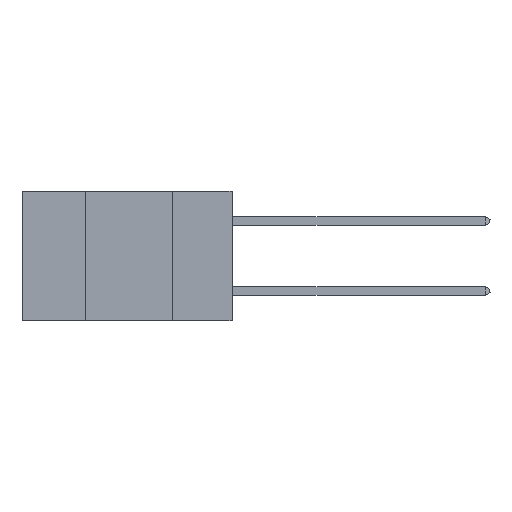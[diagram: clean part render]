
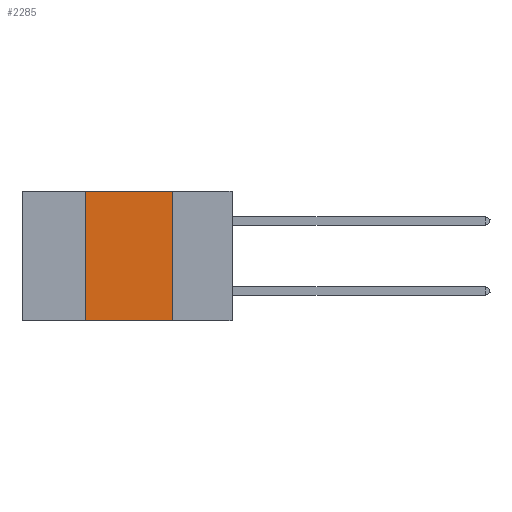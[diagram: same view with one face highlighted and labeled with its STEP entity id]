
A CAD part, left-side view. The second image highlights one B-rep face of the part: STEP entity #2285.
In plain terms, the highlighted planar face has unit normal (-1, 0, 0).
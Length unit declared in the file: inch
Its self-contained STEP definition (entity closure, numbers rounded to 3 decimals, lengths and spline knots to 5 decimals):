
#18 = CARTESIAN_POINT ( 'NONE',  ( 0., 0.6, -0.37 ) ) ;
#862 = DIRECTION ( 'NONE',  ( 0., 0., -1. ) ) ;
#1219 = FACE_OUTER_BOUND ( 'NONE', #6404, .T. ) ;
#1738 = CARTESIAN_POINT ( 'NONE',  ( 0., 0.42, -0.37 ) ) ;
#2285 = ADVANCED_FACE ( 'NONE', ( #1219 ), #3434, .F. ) ;
#2644 = EDGE_CURVE ( 'NONE', #15117, #19382, #21342, .T. ) ;
#2808 = VECTOR ( 'NONE', #862, 39.37008 ) ;
#3316 = LINE ( 'NONE', #18, #18737 ) ;
#3434 = PLANE ( 'NONE',  #4460 ) ;
#4152 = VERTEX_POINT ( 'NONE', #21878 ) ;
#4460 = AXIS2_PLACEMENT_3D ( 'NONE', #15384, #17049, #6880 ) ;
#5957 = ORIENTED_EDGE ( 'NONE', *, *, #6085, .T. ) ;
#6085 = EDGE_CURVE ( 'NONE', #17109, #19382, #3316, .T. ) ;
#6404 = EDGE_LOOP ( 'NONE', ( #21267, #8382, #13444, #5957 ) ) ;
#6756 = VECTOR ( 'NONE', #12698, 39.37008 ) ;
#6880 = DIRECTION ( 'NONE',  ( 0., 0., -1. ) ) ;
#7506 = EDGE_CURVE ( 'NONE', #4152, #15117, #16346, .T. ) ;
#7610 = CARTESIAN_POINT ( 'NONE',  ( 0., 0.6, 0. ) ) ;
#8083 = CARTESIAN_POINT ( 'NONE',  ( 0., 0.17, -0.37 ) ) ;
#8382 = ORIENTED_EDGE ( 'NONE', *, *, #7506, .F. ) ;
#9545 = DIRECTION ( 'NONE',  ( 0., 0., 1. ) ) ;
#12006 = DIRECTION ( 'NONE',  ( 0., -1., 0. ) ) ;
#12698 = DIRECTION ( 'NONE',  ( 0., -1., 0. ) ) ;
#13444 = ORIENTED_EDGE ( 'NONE', *, *, #21210, .F. ) ;
#15117 = VERTEX_POINT ( 'NONE', #16365 ) ;
#15166 = VECTOR ( 'NONE', #9545, 39.37008 ) ;
#15384 = CARTESIAN_POINT ( 'NONE',  ( 0., 0.6, 0. ) ) ;
#16346 = LINE ( 'NONE', #7610, #6756 ) ;
#16365 = CARTESIAN_POINT ( 'NONE',  ( 0., 0.17, 0. ) ) ;
#17049 = DIRECTION ( 'NONE',  ( 1., 0., 0. ) ) ;
#17109 = VERTEX_POINT ( 'NONE', #1738 ) ;
#18737 = VECTOR ( 'NONE', #12006, 39.37008 ) ;
#19382 = VERTEX_POINT ( 'NONE', #8083 ) ;
#19533 = CARTESIAN_POINT ( 'NONE',  ( 0., 0.17, 0. ) ) ;
#19655 = CARTESIAN_POINT ( 'NONE',  ( 0., 0.42, 0. ) ) ;
#20101 = LINE ( 'NONE', #19655, #15166 ) ;
#21210 = EDGE_CURVE ( 'NONE', #17109, #4152, #20101, .T. ) ;
#21267 = ORIENTED_EDGE ( 'NONE', *, *, #2644, .F. ) ;
#21342 = LINE ( 'NONE', #19533, #2808 ) ;
#21878 = CARTESIAN_POINT ( 'NONE',  ( 0., 0.42, 0. ) ) ;
